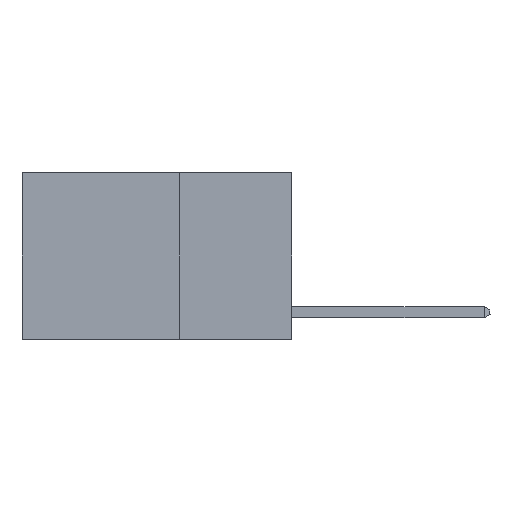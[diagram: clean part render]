
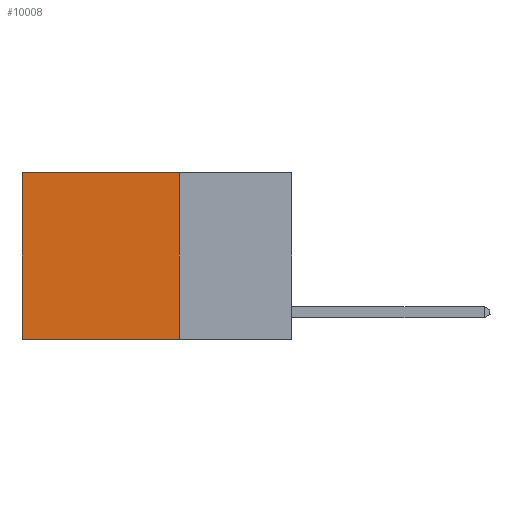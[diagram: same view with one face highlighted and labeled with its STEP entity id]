
A CAD part, left-side view. The second image highlights one B-rep face of the part: STEP entity #10008.
In plain terms, the highlighted planar face has unit normal (-1, 0, 0).
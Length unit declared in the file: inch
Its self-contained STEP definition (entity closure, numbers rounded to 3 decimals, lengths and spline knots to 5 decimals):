
#139 = VECTOR ( 'NONE', #3413, 39.37008 ) ;
#970 = VERTEX_POINT ( 'NONE', #8528 ) ;
#1113 = CARTESIAN_POINT ( 'NONE',  ( 0.2625, 0.6, 0. ) ) ;
#1873 = VECTOR ( 'NONE', #2552, 39.37008 ) ;
#2280 = ORIENTED_EDGE ( 'NONE', *, *, #5132, .T. ) ;
#2552 = DIRECTION ( 'NONE',  ( 0., 1., 0. ) ) ;
#2718 = FACE_OUTER_BOUND ( 'NONE', #6085, .T. ) ;
#2922 = CARTESIAN_POINT ( 'NONE',  ( 0.2625, 0.6, 0. ) ) ;
#3128 = DIRECTION ( 'NONE',  ( 0., 0., -1. ) ) ;
#3292 = ORIENTED_EDGE ( 'NONE', *, *, #8943, .F. ) ;
#3413 = DIRECTION ( 'NONE',  ( 0., 1., 0. ) ) ;
#3504 = DIRECTION ( 'NONE',  ( 0., 0., -1. ) ) ;
#3505 = DIRECTION ( 'NONE',  ( 0., 0., -1. ) ) ;
#4900 = CARTESIAN_POINT ( 'NONE',  ( 0.2625, 0.25, 0. ) ) ;
#5132 = EDGE_CURVE ( 'NONE', #970, #10029, #8271, .T. ) ;
#5206 = EDGE_CURVE ( 'NONE', #970, #9908, #8924, .T. ) ;
#5426 = CARTESIAN_POINT ( 'NONE',  ( 0.2625, 0.25, -0.37 ) ) ;
#5743 = CARTESIAN_POINT ( 'NONE',  ( 0.2625, 0.25, 0. ) ) ;
#5852 = DIRECTION ( 'NONE',  ( 1., 0., 0. ) ) ;
#6085 = EDGE_LOOP ( 'NONE', ( #6368, #3292, #7880, #2280 ) ) ;
#6271 = VERTEX_POINT ( 'NONE', #9539 ) ;
#6368 = ORIENTED_EDGE ( 'NONE', *, *, #9495, .T. ) ;
#6559 = PLANE ( 'NONE',  #10028 ) ;
#7166 = LINE ( 'NONE', #2922, #7300 ) ;
#7300 = VECTOR ( 'NONE', #3128, 39.37008 ) ;
#7362 = CARTESIAN_POINT ( 'NONE',  ( 0.2625, 0.25, -0.37 ) ) ;
#7880 = ORIENTED_EDGE ( 'NONE', *, *, #5206, .F. ) ;
#8271 = LINE ( 'NONE', #9631, #1873 ) ;
#8528 = CARTESIAN_POINT ( 'NONE',  ( 0.2625, 0.25, 0. ) ) ;
#8837 = LINE ( 'NONE', #7362, #139 ) ;
#8924 = LINE ( 'NONE', #4900, #9643 ) ;
#8943 = EDGE_CURVE ( 'NONE', #9908, #6271, #8837, .T. ) ;
#9495 = EDGE_CURVE ( 'NONE', #10029, #6271, #7166, .T. ) ;
#9539 = CARTESIAN_POINT ( 'NONE',  ( 0.2625, 0.6, -0.37 ) ) ;
#9631 = CARTESIAN_POINT ( 'NONE',  ( 0.2625, 0.25, 0. ) ) ;
#9643 = VECTOR ( 'NONE', #3504, 39.37008 ) ;
#9908 = VERTEX_POINT ( 'NONE', #5426 ) ;
#10008 = ADVANCED_FACE ( 'NONE', ( #2718 ), #6559, .F. ) ;
#10028 = AXIS2_PLACEMENT_3D ( 'NONE', #5743, #5852, #3505 ) ;
#10029 = VERTEX_POINT ( 'NONE', #1113 ) ;
